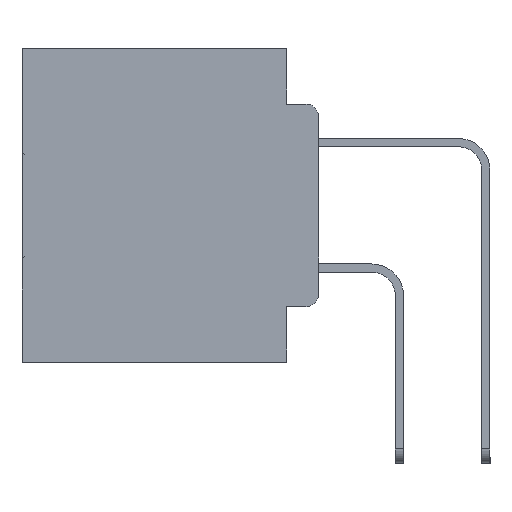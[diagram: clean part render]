
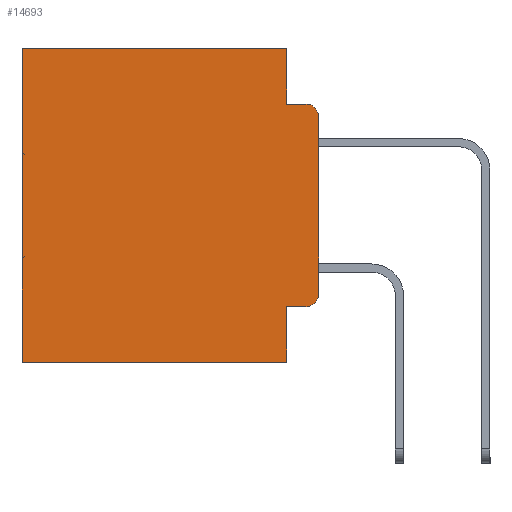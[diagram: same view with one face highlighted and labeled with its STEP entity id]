
A CAD part, left-side view. The second image highlights one B-rep face of the part: STEP entity #14693.
In plain terms, the highlighted planar face has unit normal (-1, 0, 0).
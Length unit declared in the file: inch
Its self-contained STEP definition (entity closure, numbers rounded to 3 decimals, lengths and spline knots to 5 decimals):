
#271 = CARTESIAN_POINT ( 'NONE',  ( 0.298, 0., 0. ) ) ;
#463 = CARTESIAN_POINT ( 'NONE',  ( 0.298, 0.473, 0. ) ) ;
#522 = DIRECTION ( 'NONE',  ( 0., 0., -1. ) ) ;
#548 = LINE ( 'NONE', #27732, #5991 ) ;
#728 = VECTOR ( 'NONE', #3165, 39.37008 ) ;
#1074 = DIRECTION ( 'NONE',  ( 0., 1., 0. ) ) ;
#1969 = EDGE_CURVE ( 'NONE', #25572, #4936, #31554, .T. ) ;
#2147 = CARTESIAN_POINT ( 'NONE',  ( 0.298, 0.051, 0. ) ) ;
#2615 = EDGE_CURVE ( 'NONE', #25572, #21482, #11605, .T. ) ;
#2916 = CARTESIAN_POINT ( 'NONE',  ( 0.298, 0., -0.1085 ) ) ;
#3165 = DIRECTION ( 'NONE',  ( 0., 0., -1. ) ) ;
#3178 = CARTESIAN_POINT ( 'NONE',  ( 0.298, 0.02, -0.0885 ) ) ;
#3562 = EDGE_CURVE ( 'NONE', #9718, #23909, #25774, .T. ) ;
#3671 = VECTOR ( 'NONE', #522, 39.37008 ) ;
#4936 = VERTEX_POINT ( 'NONE', #29210 ) ;
#5147 = AXIS2_PLACEMENT_3D ( 'NONE', #29899, #14012, #32475 ) ;
#5506 = ORIENTED_EDGE ( 'NONE', *, *, #22792, .F. ) ;
#5991 = VECTOR ( 'NONE', #1074, 39.37008 ) ;
#7643 = VERTEX_POINT ( 'NONE', #9861 ) ;
#7759 = LINE ( 'NONE', #9253, #21124 ) ;
#7947 = ORIENTED_EDGE ( 'NONE', *, *, #3562, .F. ) ;
#8145 = VECTOR ( 'NONE', #9254, 39.37008 ) ;
#8174 = CIRCLE ( 'NONE', #10598, 0.02 ) ;
#9142 = CARTESIAN_POINT ( 'NONE',  ( 0.298, 0.051, -0.0885 ) ) ;
#9253 = CARTESIAN_POINT ( 'NONE',  ( 0.298, 0., 0. ) ) ;
#9254 = DIRECTION ( 'NONE',  ( 0., -1., 0. ) ) ;
#9553 = CARTESIAN_POINT ( 'NONE',  ( 0.298, 0., -0.3915 ) ) ;
#9636 = ORIENTED_EDGE ( 'NONE', *, *, #2615, .T. ) ;
#9718 = VERTEX_POINT ( 'NONE', #2916 ) ;
#9861 = CARTESIAN_POINT ( 'NONE',  ( 0.298, 0.051, 0. ) ) ;
#10137 = DIRECTION ( 'NONE',  ( 0., 0., -1. ) ) ;
#10598 = AXIS2_PLACEMENT_3D ( 'NONE', #10797, #29387, #13481 ) ;
#10764 = VECTOR ( 'NONE', #12087, 39.37008 ) ;
#10797 = CARTESIAN_POINT ( 'NONE',  ( 0.298, 0.02, -0.3915 ) ) ;
#11524 = EDGE_CURVE ( 'NONE', #21482, #23909, #8174, .T. ) ;
#11605 = LINE ( 'NONE', #32327, #10764 ) ;
#11668 = CARTESIAN_POINT ( 'NONE',  ( 0.298, 0.473, 0. ) ) ;
#11940 = DIRECTION ( 'NONE',  ( 0., 1., 0. ) ) ;
#11984 = EDGE_CURVE ( 'NONE', #33841, #22625, #15241, .T. ) ;
#12087 = DIRECTION ( 'NONE',  ( 0., -1., 0. ) ) ;
#12216 = EDGE_LOOP ( 'NONE', ( #7947, #22173, #30784, #28747, #16329, #30406, #5506, #28371, #9636, #24689 ) ) ;
#12294 = CIRCLE ( 'NONE', #5147, 0.02 ) ;
#12540 = DIRECTION ( 'NONE',  ( 1., 0., 0. ) ) ;
#13481 = DIRECTION ( 'NONE',  ( 0., 0., -1. ) ) ;
#14012 = DIRECTION ( 'NONE',  ( -1., 0., 0. ) ) ;
#14528 = CARTESIAN_POINT ( 'NONE',  ( 0.298, 0.02, -0.4115 ) ) ;
#14693 = ADVANCED_FACE ( 'NONE', ( #33908 ), #28358, .F. ) ;
#15026 = LINE ( 'NONE', #2147, #22975 ) ;
#15089 = VERTEX_POINT ( 'NONE', #30044 ) ;
#15241 = LINE ( 'NONE', #9142, #8145 ) ;
#15534 = CARTESIAN_POINT ( 'NONE',  ( 0.298, 0.051, -0.0885 ) ) ;
#16238 = EDGE_CURVE ( 'NONE', #25665, #15089, #29829, .T. ) ;
#16329 = ORIENTED_EDGE ( 'NONE', *, *, #27557, .T. ) ;
#21124 = VECTOR ( 'NONE', #11940, 39.37008 ) ;
#21482 = VERTEX_POINT ( 'NONE', #14528 ) ;
#22173 = ORIENTED_EDGE ( 'NONE', *, *, #28056, .T. ) ;
#22625 = VERTEX_POINT ( 'NONE', #3178 ) ;
#22792 = EDGE_CURVE ( 'NONE', #4936, #15089, #548, .T. ) ;
#22975 = VECTOR ( 'NONE', #10137, 39.37008 ) ;
#23784 = VECTOR ( 'NONE', #30106, 39.37008 ) ;
#23909 = VERTEX_POINT ( 'NONE', #9553 ) ;
#24689 = ORIENTED_EDGE ( 'NONE', *, *, #11524, .T. ) ;
#25572 = VERTEX_POINT ( 'NONE', #32489 ) ;
#25665 = VERTEX_POINT ( 'NONE', #11668 ) ;
#25774 = LINE ( 'NONE', #271, #3671 ) ;
#27557 = EDGE_CURVE ( 'NONE', #7643, #25665, #7759, .T. ) ;
#27732 = CARTESIAN_POINT ( 'NONE',  ( 0.298, 0., -0.5 ) ) ;
#28056 = EDGE_CURVE ( 'NONE', #9718, #22625, #12294, .T. ) ;
#28358 = PLANE ( 'NONE',  #30037 ) ;
#28371 = ORIENTED_EDGE ( 'NONE', *, *, #1969, .F. ) ;
#28747 = ORIENTED_EDGE ( 'NONE', *, *, #33831, .F. ) ;
#29210 = CARTESIAN_POINT ( 'NONE',  ( 0.298, 0.051, -0.5 ) ) ;
#29387 = DIRECTION ( 'NONE',  ( -1., 0., 0. ) ) ;
#29829 = LINE ( 'NONE', #463, #728 ) ;
#29899 = CARTESIAN_POINT ( 'NONE',  ( 0.298, 0.02, -0.1085 ) ) ;
#30037 = AXIS2_PLACEMENT_3D ( 'NONE', #30968, #12540, #31077 ) ;
#30044 = CARTESIAN_POINT ( 'NONE',  ( 0.298, 0.473, -0.5 ) ) ;
#30106 = DIRECTION ( 'NONE',  ( 0., 0., -1. ) ) ;
#30406 = ORIENTED_EDGE ( 'NONE', *, *, #16238, .T. ) ;
#30784 = ORIENTED_EDGE ( 'NONE', *, *, #11984, .F. ) ;
#30968 = CARTESIAN_POINT ( 'NONE',  ( 0.298, 0., 0. ) ) ;
#31077 = DIRECTION ( 'NONE',  ( 0., 0., -1. ) ) ;
#31193 = CARTESIAN_POINT ( 'NONE',  ( 0.298, 0.051, 0. ) ) ;
#31554 = LINE ( 'NONE', #31193, #23784 ) ;
#32327 = CARTESIAN_POINT ( 'NONE',  ( 0.298, 0.051, -0.4115 ) ) ;
#32475 = DIRECTION ( 'NONE',  ( 0., 0., -1. ) ) ;
#32489 = CARTESIAN_POINT ( 'NONE',  ( 0.298, 0.051, -0.4115 ) ) ;
#33831 = EDGE_CURVE ( 'NONE', #7643, #33841, #15026, .T. ) ;
#33841 = VERTEX_POINT ( 'NONE', #15534 ) ;
#33908 = FACE_OUTER_BOUND ( 'NONE', #12216, .T. ) ;
